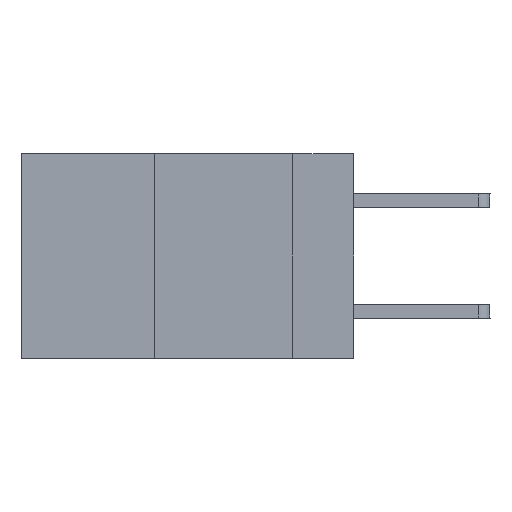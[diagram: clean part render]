
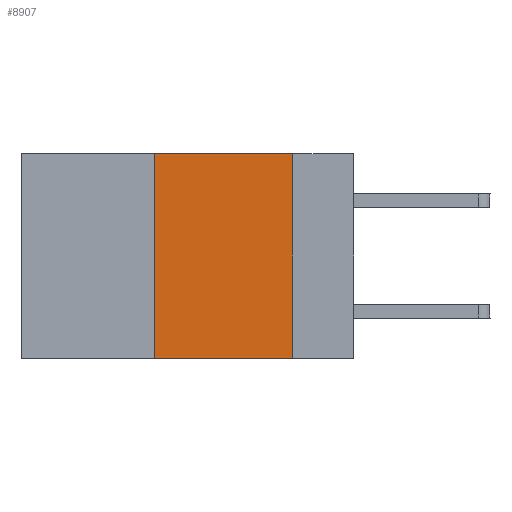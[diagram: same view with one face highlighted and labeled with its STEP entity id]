
A CAD part, left-side view. The second image highlights one B-rep face of the part: STEP entity #8907.
In plain terms, the highlighted planar face has unit normal (-1, 0, 0).
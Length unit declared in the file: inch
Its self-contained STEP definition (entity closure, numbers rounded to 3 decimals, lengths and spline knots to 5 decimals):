
#59 = DIRECTION ( 'NONE',  ( 0., -1., 0. ) ) ;
#422 = DIRECTION ( 'NONE',  ( 0., 0., -1. ) ) ;
#925 = VECTOR ( 'NONE', #6949, 39.37008 ) ;
#948 = ORIENTED_EDGE ( 'NONE', *, *, #11641, .T. ) ;
#1167 = DIRECTION ( 'NONE',  ( 0., -1., 0. ) ) ;
#1431 = FACE_OUTER_BOUND ( 'NONE', #11649, .T. ) ;
#1476 = CARTESIAN_POINT ( 'NONE',  ( 0., 0.36, -0.37 ) ) ;
#1527 = CARTESIAN_POINT ( 'NONE',  ( 0., 0.36, 0. ) ) ;
#1696 = EDGE_CURVE ( 'NONE', #3828, #3102, #8188, .T. ) ;
#1811 = CARTESIAN_POINT ( 'NONE',  ( 0., 0.6, 0. ) ) ;
#3102 = VERTEX_POINT ( 'NONE', #11586 ) ;
#3124 = CARTESIAN_POINT ( 'NONE',  ( 0., 0.36, 0. ) ) ;
#3607 = CARTESIAN_POINT ( 'NONE',  ( 0., 0.11, -0.37 ) ) ;
#3621 = LINE ( 'NONE', #1527, #5114 ) ;
#3745 = EDGE_CURVE ( 'NONE', #3102, #8396, #7963, .T. ) ;
#3828 = VERTEX_POINT ( 'NONE', #3124 ) ;
#4239 = CARTESIAN_POINT ( 'NONE',  ( 0., 0.6, 0. ) ) ;
#4684 = VERTEX_POINT ( 'NONE', #1476 ) ;
#4900 = ORIENTED_EDGE ( 'NONE', *, *, #3745, .F. ) ;
#5114 = VECTOR ( 'NONE', #7707, 39.37008 ) ;
#5135 = CARTESIAN_POINT ( 'NONE',  ( 0., 0.6, -0.37 ) ) ;
#6241 = VECTOR ( 'NONE', #59, 39.37008 ) ;
#6949 = DIRECTION ( 'NONE',  ( 0., 0., -1. ) ) ;
#6996 = VECTOR ( 'NONE', #1167, 39.37008 ) ;
#7202 = ORIENTED_EDGE ( 'NONE', *, *, #1696, .F. ) ;
#7280 = LINE ( 'NONE', #5135, #6996 ) ;
#7707 = DIRECTION ( 'NONE',  ( 0., 0., 1. ) ) ;
#7963 = LINE ( 'NONE', #12079, #925 ) ;
#8188 = LINE ( 'NONE', #4239, #6241 ) ;
#8396 = VERTEX_POINT ( 'NONE', #3607 ) ;
#8487 = ORIENTED_EDGE ( 'NONE', *, *, #13164, .F. ) ;
#8695 = AXIS2_PLACEMENT_3D ( 'NONE', #1811, #9637, #422 ) ;
#8875 = PLANE ( 'NONE',  #8695 ) ;
#8907 = ADVANCED_FACE ( 'NONE', ( #1431 ), #8875, .F. ) ;
#9637 = DIRECTION ( 'NONE',  ( 1., 0., 0. ) ) ;
#11586 = CARTESIAN_POINT ( 'NONE',  ( 0., 0.11, 0. ) ) ;
#11641 = EDGE_CURVE ( 'NONE', #4684, #8396, #7280, .T. ) ;
#11649 = EDGE_LOOP ( 'NONE', ( #4900, #7202, #8487, #948 ) ) ;
#12079 = CARTESIAN_POINT ( 'NONE',  ( 0., 0.11, 0. ) ) ;
#13164 = EDGE_CURVE ( 'NONE', #4684, #3828, #3621, .T. ) ;
